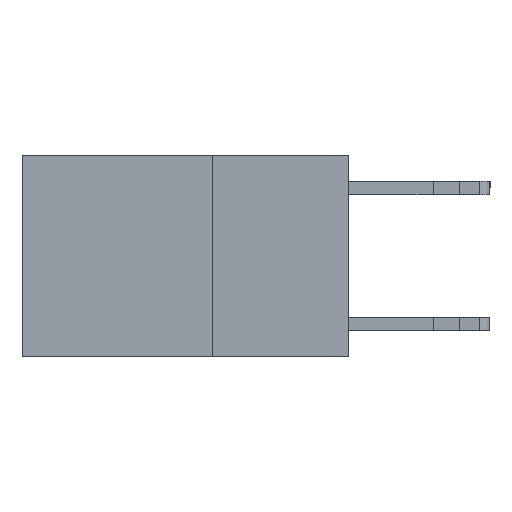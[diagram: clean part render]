
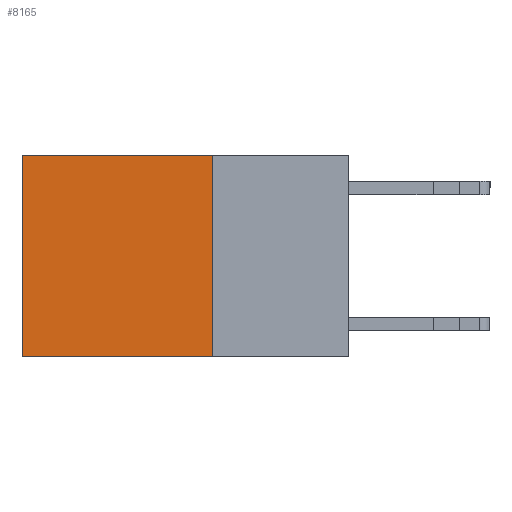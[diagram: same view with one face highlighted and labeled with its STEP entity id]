
A CAD part, left-side view. The second image highlights one B-rep face of the part: STEP entity #8165.
In plain terms, the highlighted planar face has unit normal (-1, 0, 0).
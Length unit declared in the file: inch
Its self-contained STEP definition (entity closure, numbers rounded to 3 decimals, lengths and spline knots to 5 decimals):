
#293 = EDGE_CURVE ( 'NONE', #3849, #4668, #17559, .T. ) ;
#891 = DIRECTION ( 'NONE',  ( 1., 0., 0. ) ) ;
#2294 = EDGE_CURVE ( 'NONE', #3849, #10499, #25110, .T. ) ;
#2309 = DIRECTION ( 'NONE',  ( 0., 0., -1. ) ) ;
#2585 = ORIENTED_EDGE ( 'NONE', *, *, #293, .T. ) ;
#3021 = DIRECTION ( 'NONE',  ( 0., 1., 0. ) ) ;
#3849 = VERTEX_POINT ( 'NONE', #15314 ) ;
#4283 = CARTESIAN_POINT ( 'NONE',  ( 0.2625, 0.25, 0. ) ) ;
#4668 = VERTEX_POINT ( 'NONE', #16648 ) ;
#4726 = ORIENTED_EDGE ( 'NONE', *, *, #2294, .F. ) ;
#6155 = CARTESIAN_POINT ( 'NONE',  ( 0.2625, 0.6, -0.37 ) ) ;
#8165 = ADVANCED_FACE ( 'NONE', ( #24585 ), #12491, .F. ) ;
#9400 = CARTESIAN_POINT ( 'NONE',  ( 0.2625, 0.25, 0. ) ) ;
#10499 = VERTEX_POINT ( 'NONE', #25256 ) ;
#10948 = DIRECTION ( 'NONE',  ( 0., 0., -1. ) ) ;
#11378 = ORIENTED_EDGE ( 'NONE', *, *, #22646, .F. ) ;
#11452 = AXIS2_PLACEMENT_3D ( 'NONE', #14915, #891, #20335 ) ;
#12491 = PLANE ( 'NONE',  #11452 ) ;
#12940 = CARTESIAN_POINT ( 'NONE',  ( 0.2625, 0.25, -0.37 ) ) ;
#13105 = VECTOR ( 'NONE', #2309, 39.37008 ) ;
#14915 = CARTESIAN_POINT ( 'NONE',  ( 0.2625, 0.25, 0. ) ) ;
#15314 = CARTESIAN_POINT ( 'NONE',  ( 0.2625, 0.25, 0. ) ) ;
#15942 = LINE ( 'NONE', #19934, #13105 ) ;
#16648 = CARTESIAN_POINT ( 'NONE',  ( 0.2625, 0.6, 0. ) ) ;
#16947 = VECTOR ( 'NONE', #3021, 39.37008 ) ;
#17144 = EDGE_CURVE ( 'NONE', #4668, #25106, #15942, .T. ) ;
#17559 = LINE ( 'NONE', #4283, #18174 ) ;
#18174 = VECTOR ( 'NONE', #23609, 39.37008 ) ;
#18209 = ORIENTED_EDGE ( 'NONE', *, *, #17144, .T. ) ;
#19934 = CARTESIAN_POINT ( 'NONE',  ( 0.2625, 0.6, 0. ) ) ;
#20335 = DIRECTION ( 'NONE',  ( 0., 0., -1. ) ) ;
#21410 = EDGE_LOOP ( 'NONE', ( #18209, #11378, #4726, #2585 ) ) ;
#22646 = EDGE_CURVE ( 'NONE', #10499, #25106, #24906, .T. ) ;
#22967 = VECTOR ( 'NONE', #10948, 39.37008 ) ;
#23609 = DIRECTION ( 'NONE',  ( 0., 1., 0. ) ) ;
#24585 = FACE_OUTER_BOUND ( 'NONE', #21410, .T. ) ;
#24906 = LINE ( 'NONE', #12940, #16947 ) ;
#25106 = VERTEX_POINT ( 'NONE', #6155 ) ;
#25110 = LINE ( 'NONE', #9400, #22967 ) ;
#25256 = CARTESIAN_POINT ( 'NONE',  ( 0.2625, 0.25, -0.37 ) ) ;
